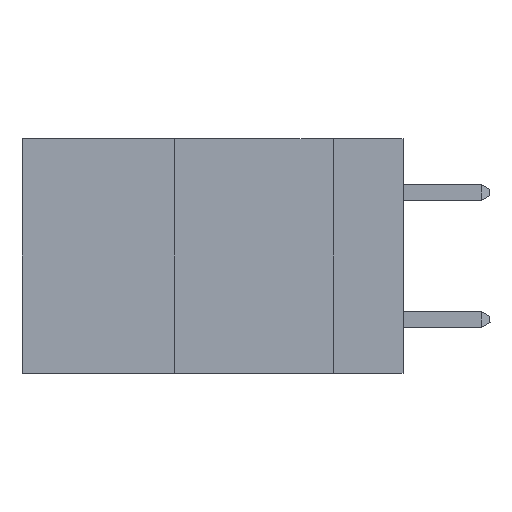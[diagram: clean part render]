
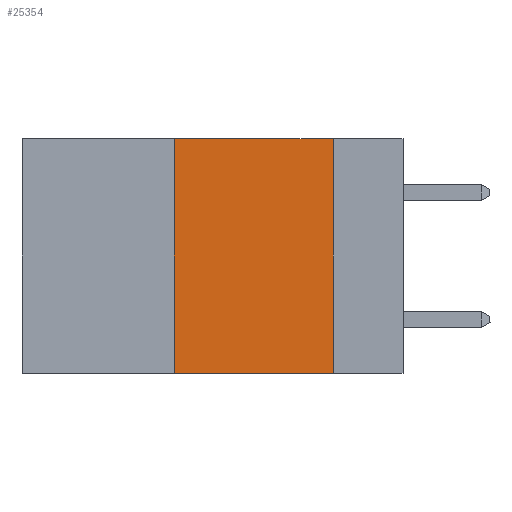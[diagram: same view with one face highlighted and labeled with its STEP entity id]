
A CAD part, left-side view. The second image highlights one B-rep face of the part: STEP entity #25354.
In plain terms, the highlighted planar face has unit normal (-1, 0, 0).
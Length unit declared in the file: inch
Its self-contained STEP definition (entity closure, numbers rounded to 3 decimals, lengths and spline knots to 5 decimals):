
#1032 = EDGE_CURVE ( 'NONE', #28973, #4712, #13696, .T. ) ;
#1108 = ORIENTED_EDGE ( 'NONE', *, *, #16582, .F. ) ;
#2578 = VECTOR ( 'NONE', #33546, 39.37008 ) ;
#3287 = EDGE_CURVE ( 'NONE', #29918, #7442, #9994, .T. ) ;
#4712 = VERTEX_POINT ( 'NONE', #16490 ) ;
#7442 = VERTEX_POINT ( 'NONE', #27464 ) ;
#7453 = ORIENTED_EDGE ( 'NONE', *, *, #34585, .F. ) ;
#9189 = CARTESIAN_POINT ( 'NONE',  ( 0., 0.36, -0.37 ) ) ;
#9795 = ORIENTED_EDGE ( 'NONE', *, *, #1032, .F. ) ;
#9832 = ORIENTED_EDGE ( 'NONE', *, *, #3287, .T. ) ;
#9994 = LINE ( 'NONE', #12301, #33645 ) ;
#12301 = CARTESIAN_POINT ( 'NONE',  ( 0., 0.6, -0.37 ) ) ;
#13696 = LINE ( 'NONE', #24659, #28274 ) ;
#13757 = EDGE_LOOP ( 'NONE', ( #7453, #9795, #1108, #9832 ) ) ;
#15273 = AXIS2_PLACEMENT_3D ( 'NONE', #32092, #32460, #24773 ) ;
#16490 = CARTESIAN_POINT ( 'NONE',  ( 0., 0.11, 0. ) ) ;
#16582 = EDGE_CURVE ( 'NONE', #29918, #28973, #33530, .T. ) ;
#17610 = PLANE ( 'NONE',  #15273 ) ;
#18232 = CARTESIAN_POINT ( 'NONE',  ( 0., 0.36, 0. ) ) ;
#18358 = DIRECTION ( 'NONE',  ( 0., 0., -1. ) ) ;
#19866 = CARTESIAN_POINT ( 'NONE',  ( 0., 0.36, 0. ) ) ;
#22365 = DIRECTION ( 'NONE',  ( 0., -1., 0. ) ) ;
#22892 = LINE ( 'NONE', #32922, #27479 ) ;
#24659 = CARTESIAN_POINT ( 'NONE',  ( 0., 0.6, 0. ) ) ;
#24773 = DIRECTION ( 'NONE',  ( 0., 0., -1. ) ) ;
#25354 = ADVANCED_FACE ( 'NONE', ( #25504 ), #17610, .F. ) ;
#25504 = FACE_OUTER_BOUND ( 'NONE', #13757, .T. ) ;
#27464 = CARTESIAN_POINT ( 'NONE',  ( 0., 0.11, -0.37 ) ) ;
#27479 = VECTOR ( 'NONE', #18358, 39.37008 ) ;
#28274 = VECTOR ( 'NONE', #22365, 39.37008 ) ;
#28973 = VERTEX_POINT ( 'NONE', #19866 ) ;
#29918 = VERTEX_POINT ( 'NONE', #9189 ) ;
#32092 = CARTESIAN_POINT ( 'NONE',  ( 0., 0.6, 0. ) ) ;
#32460 = DIRECTION ( 'NONE',  ( 1., 0., 0. ) ) ;
#32922 = CARTESIAN_POINT ( 'NONE',  ( 0., 0.11, 0. ) ) ;
#33530 = LINE ( 'NONE', #18232, #2578 ) ;
#33546 = DIRECTION ( 'NONE',  ( 0., 0., 1. ) ) ;
#33645 = VECTOR ( 'NONE', #35423, 39.37008 ) ;
#34585 = EDGE_CURVE ( 'NONE', #4712, #7442, #22892, .T. ) ;
#35423 = DIRECTION ( 'NONE',  ( 0., -1., 0. ) ) ;
